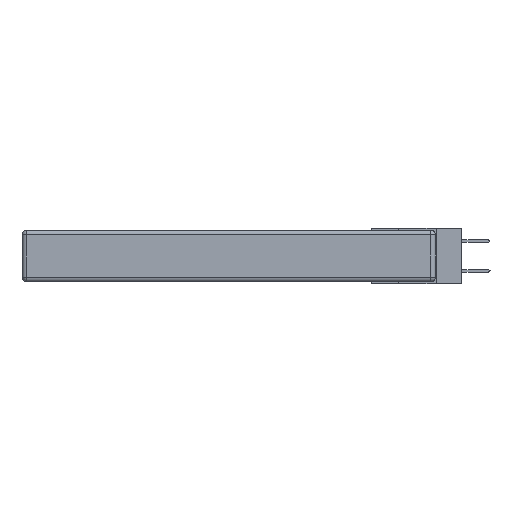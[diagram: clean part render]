
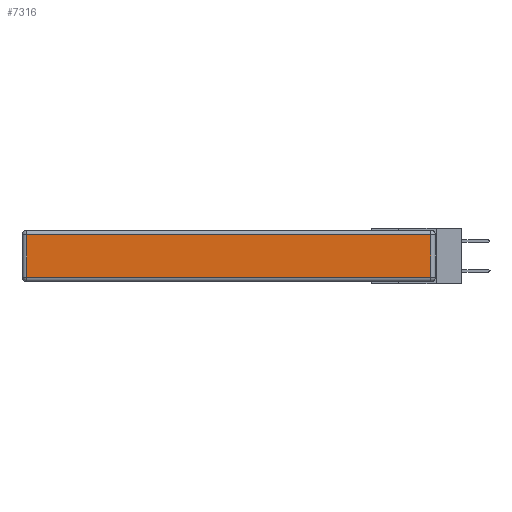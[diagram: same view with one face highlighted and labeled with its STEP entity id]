
A CAD part, left-side view. The second image highlights one B-rep face of the part: STEP entity #7316.
In plain terms, the highlighted planar face has unit normal (-1, 0, 0).
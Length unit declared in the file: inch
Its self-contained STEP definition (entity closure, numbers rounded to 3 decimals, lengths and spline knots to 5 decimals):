
#32 = VECTOR ( 'NONE', #1775, 39.37008 ) ;
#986 = CARTESIAN_POINT ( 'NONE',  ( 0., 0.03, -0.313 ) ) ;
#1588 = CARTESIAN_POINT ( 'NONE',  ( 0., 2.72, -0.343 ) ) ;
#1775 = DIRECTION ( 'NONE',  ( 0., -1., 0. ) ) ;
#2055 = DIRECTION ( 'NONE',  ( -1., 0., 0. ) ) ;
#2132 = LINE ( 'NONE', #22766, #9779 ) ;
#2869 = DIRECTION ( 'NONE',  ( 0., 0., 1. ) ) ;
#3303 = FACE_OUTER_BOUND ( 'NONE', #18802, .T. ) ;
#4818 = CARTESIAN_POINT ( 'NONE',  ( 0., 0.03, -0.343 ) ) ;
#6680 = ORIENTED_EDGE ( 'NONE', *, *, #11240, .T. ) ;
#6833 = ORIENTED_EDGE ( 'NONE', *, *, #15432, .T. ) ;
#7094 = VECTOR ( 'NONE', #14186, 39.37008 ) ;
#7316 = ADVANCED_FACE ( 'NONE', ( #3303 ), #21013, .T. ) ;
#7433 = CARTESIAN_POINT ( 'NONE',  ( 0., 0.03, -0.03 ) ) ;
#7437 = LINE ( 'NONE', #4818, #20690 ) ;
#7485 = DIRECTION ( 'NONE',  ( 0., 0., 1. ) ) ;
#9779 = VECTOR ( 'NONE', #13761, 39.37008 ) ;
#10500 = LINE ( 'NONE', #1588, #7094 ) ;
#11240 = EDGE_CURVE ( 'NONE', #15615, #12843, #7437, .T. ) ;
#11316 = ORIENTED_EDGE ( 'NONE', *, *, #20776, .T. ) ;
#12460 = VERTEX_POINT ( 'NONE', #19666 ) ;
#12489 = CARTESIAN_POINT ( 'NONE',  ( 0., 0., -0.313 ) ) ;
#12843 = VERTEX_POINT ( 'NONE', #7433 ) ;
#13761 = DIRECTION ( 'NONE',  ( 0., 1., 0. ) ) ;
#14186 = DIRECTION ( 'NONE',  ( 0., 0., -1. ) ) ;
#15086 = AXIS2_PLACEMENT_3D ( 'NONE', #15658, #2055, #7485 ) ;
#15432 = EDGE_CURVE ( 'NONE', #12460, #19679, #10500, .T. ) ;
#15615 = VERTEX_POINT ( 'NONE', #986 ) ;
#15658 = CARTESIAN_POINT ( 'NONE',  ( 0., 0., -0.343 ) ) ;
#17786 = ORIENTED_EDGE ( 'NONE', *, *, #23124, .T. ) ;
#18802 = EDGE_LOOP ( 'NONE', ( #11316, #6680, #17786, #6833 ) ) ;
#19666 = CARTESIAN_POINT ( 'NONE',  ( 0., 2.72, -0.03 ) ) ;
#19679 = VERTEX_POINT ( 'NONE', #20174 ) ;
#19764 = LINE ( 'NONE', #12489, #32 ) ;
#20174 = CARTESIAN_POINT ( 'NONE',  ( 0., 2.72, -0.313 ) ) ;
#20690 = VECTOR ( 'NONE', #2869, 39.37008 ) ;
#20776 = EDGE_CURVE ( 'NONE', #19679, #15615, #19764, .T. ) ;
#21013 = PLANE ( 'NONE',  #15086 ) ;
#22766 = CARTESIAN_POINT ( 'NONE',  ( 0., 2.75, -0.03 ) ) ;
#23124 = EDGE_CURVE ( 'NONE', #12843, #12460, #2132, .T. ) ;
